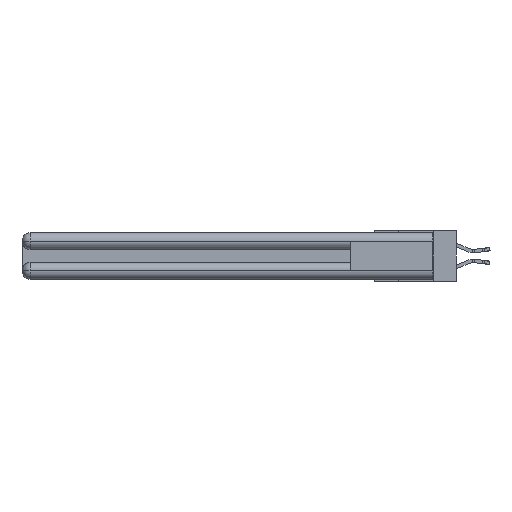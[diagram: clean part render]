
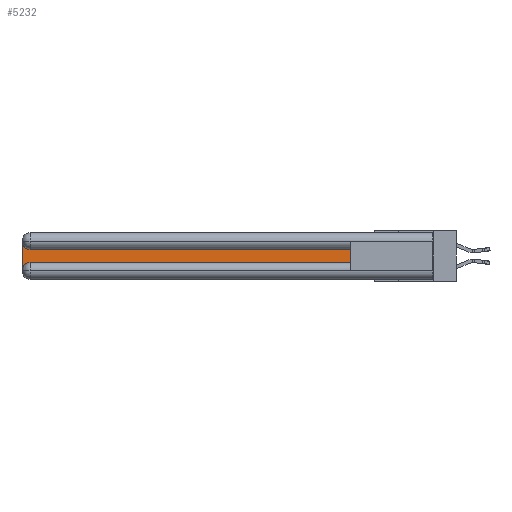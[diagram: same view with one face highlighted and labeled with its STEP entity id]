
A CAD part, left-side view. The second image highlights one B-rep face of the part: STEP entity #5232.
In plain terms, the highlighted planar face has unit normal (-1, 0, 0).
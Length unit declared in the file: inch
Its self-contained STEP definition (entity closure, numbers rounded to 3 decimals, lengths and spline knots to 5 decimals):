
#82 = CARTESIAN_POINT ( 'NONE',  ( 0.075, 2.94, -0.1225 ) ) ;
#582 = LINE ( 'NONE', #2505, #14410 ) ;
#2026 = CARTESIAN_POINT ( 'NONE',  ( 0.075, 3., -0.2175 ) ) ;
#2505 = CARTESIAN_POINT ( 'NONE',  ( 0.075, 0.6, -0.2175 ) ) ;
#2647 = ORIENTED_EDGE ( 'NONE', *, *, #27717, .T. ) ;
#2748 = DIRECTION ( 'NONE',  ( 0., -1., 0. ) ) ;
#2974 = LINE ( 'NONE', #16321, #10736 ) ;
#3175 = DIRECTION ( 'NONE',  ( 0., 0., -1. ) ) ;
#4523 = CARTESIAN_POINT ( 'NONE',  ( 0.075, 3., -0.0625 ) ) ;
#4908 = VERTEX_POINT ( 'NONE', #34571 ) ;
#5036 = ORIENTED_EDGE ( 'NONE', *, *, #32038, .T. ) ;
#5161 = DIRECTION ( 'NONE',  ( 0., 0., 1. ) ) ;
#5232 = ADVANCED_FACE ( 'NONE', ( #30340 ), #13233, .F. ) ;
#5382 = AXIS2_PLACEMENT_3D ( 'NONE', #5711, #22248, #3175 ) ;
#5711 = CARTESIAN_POINT ( 'NONE',  ( 0.075, 2.94, -0.2775 ) ) ;
#5716 = CARTESIAN_POINT ( 'NONE',  ( 0.075, 0.6, -0.2175 ) ) ;
#5859 = CARTESIAN_POINT ( 'NONE',  ( 0.075, 0.6, -0.1225 ) ) ;
#6727 = VECTOR ( 'NONE', #23641, 39.37008 ) ;
#6813 = VERTEX_POINT ( 'NONE', #5716 ) ;
#6952 = CIRCLE ( 'NONE', #21935, 0.06 ) ;
#8280 = ORIENTED_EDGE ( 'NONE', *, *, #23087, .T. ) ;
#9309 = CARTESIAN_POINT ( 'NONE',  ( 0.075, 3., -0.2775 ) ) ;
#10195 = LINE ( 'NONE', #2026, #6727 ) ;
#10736 = VECTOR ( 'NONE', #21853, 39.37008 ) ;
#11053 = EDGE_LOOP ( 'NONE', ( #5036, #2647, #13867, #31571, #15965, #8280 ) ) ;
#12497 = CIRCLE ( 'NONE', #5382, 0.06 ) ;
#13004 = EDGE_CURVE ( 'NONE', #4908, #6813, #23825, .T. ) ;
#13233 = PLANE ( 'NONE',  #29170 ) ;
#13867 = ORIENTED_EDGE ( 'NONE', *, *, #22439, .T. ) ;
#13919 = DIRECTION ( 'NONE',  ( 1., 0., 0. ) ) ;
#14080 = CARTESIAN_POINT ( 'NONE',  ( 0.075, 0.6, -0.2175 ) ) ;
#14410 = VECTOR ( 'NONE', #5161, 39.37008 ) ;
#15965 = ORIENTED_EDGE ( 'NONE', *, *, #13004, .T. ) ;
#16321 = CARTESIAN_POINT ( 'NONE',  ( 0.075, 0.6, -0.1225 ) ) ;
#16974 = DIRECTION ( 'NONE',  ( 0., 0., -1. ) ) ;
#17367 = VECTOR ( 'NONE', #2748, 39.37008 ) ;
#17412 = VERTEX_POINT ( 'NONE', #82 ) ;
#21123 = CARTESIAN_POINT ( 'NONE',  ( 0.075, 3., -0.1225 ) ) ;
#21853 = DIRECTION ( 'NONE',  ( 0., 1., 0. ) ) ;
#21935 = AXIS2_PLACEMENT_3D ( 'NONE', #30210, #13919, #16974 ) ;
#22248 = DIRECTION ( 'NONE',  ( 1., 0., 0. ) ) ;
#22439 = EDGE_CURVE ( 'NONE', #33914, #31637, #10195, .T. ) ;
#23087 = EDGE_CURVE ( 'NONE', #6813, #28115, #582, .T. ) ;
#23641 = DIRECTION ( 'NONE',  ( 0., 0., -1. ) ) ;
#23825 = LINE ( 'NONE', #14080, #17367 ) ;
#24110 = DIRECTION ( 'NONE',  ( 1., 0., 0. ) ) ;
#27717 = EDGE_CURVE ( 'NONE', #17412, #33914, #6952, .T. ) ;
#28115 = VERTEX_POINT ( 'NONE', #5859 ) ;
#28768 = EDGE_CURVE ( 'NONE', #31637, #4908, #12497, .T. ) ;
#29170 = AXIS2_PLACEMENT_3D ( 'NONE', #21123, #24110, #35239 ) ;
#30210 = CARTESIAN_POINT ( 'NONE',  ( 0.075, 2.94, -0.0625 ) ) ;
#30340 = FACE_OUTER_BOUND ( 'NONE', #11053, .T. ) ;
#31571 = ORIENTED_EDGE ( 'NONE', *, *, #28768, .T. ) ;
#31637 = VERTEX_POINT ( 'NONE', #9309 ) ;
#32038 = EDGE_CURVE ( 'NONE', #28115, #17412, #2974, .T. ) ;
#33914 = VERTEX_POINT ( 'NONE', #4523 ) ;
#34571 = CARTESIAN_POINT ( 'NONE',  ( 0.075, 2.94, -0.2175 ) ) ;
#35239 = DIRECTION ( 'NONE',  ( 0., 0., -1. ) ) ;
